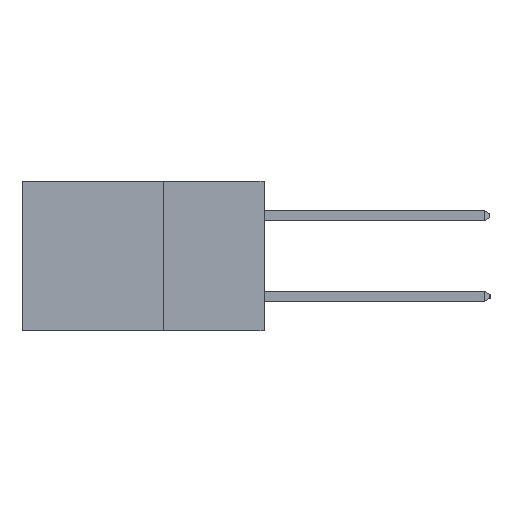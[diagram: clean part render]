
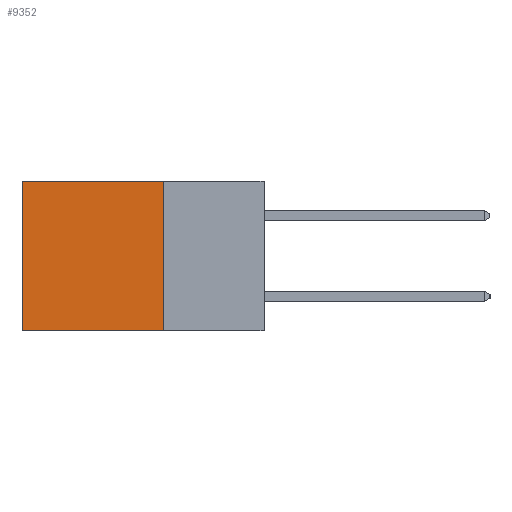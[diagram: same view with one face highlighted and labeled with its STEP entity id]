
A CAD part, left-side view. The second image highlights one B-rep face of the part: STEP entity #9352.
In plain terms, the highlighted planar face has unit normal (-1, 0, 0).
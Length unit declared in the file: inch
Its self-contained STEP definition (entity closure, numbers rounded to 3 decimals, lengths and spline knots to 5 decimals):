
#317 = FACE_OUTER_BOUND ( 'NONE', #8357, .T. ) ;
#375 = VERTEX_POINT ( 'NONE', #10325 ) ;
#2119 = DIRECTION ( 'NONE',  ( 0., 0., -1. ) ) ;
#2528 = CARTESIAN_POINT ( 'NONE',  ( 0.2615, 0.6, 0. ) ) ;
#2644 = AXIS2_PLACEMENT_3D ( 'NONE', #24282, #14203, #2119 ) ;
#3995 = VECTOR ( 'NONE', #12560, 39.37008 ) ;
#4110 = CARTESIAN_POINT ( 'NONE',  ( 0.2615, 0.25, -0.37 ) ) ;
#4550 = CARTESIAN_POINT ( 'NONE',  ( 0.2615, 0.25, 0. ) ) ;
#4869 = CARTESIAN_POINT ( 'NONE',  ( 0.2615, 0.6, -0.37 ) ) ;
#5446 = DIRECTION ( 'NONE',  ( 0., 0., -1. ) ) ;
#7671 = VECTOR ( 'NONE', #8162, 39.37008 ) ;
#7689 = ORIENTED_EDGE ( 'NONE', *, *, #18068, .F. ) ;
#7839 = EDGE_CURVE ( 'NONE', #10593, #375, #9635, .T. ) ;
#8162 = DIRECTION ( 'NONE',  ( 0., 1., 0. ) ) ;
#8357 = EDGE_LOOP ( 'NONE', ( #16962, #7689, #9791, #23721 ) ) ;
#9352 = ADVANCED_FACE ( 'NONE', ( #317 ), #10147, .F. ) ;
#9635 = LINE ( 'NONE', #19548, #15001 ) ;
#9791 = ORIENTED_EDGE ( 'NONE', *, *, #7839, .F. ) ;
#10147 = PLANE ( 'NONE',  #2644 ) ;
#10325 = CARTESIAN_POINT ( 'NONE',  ( 0.2615, 0.25, -0.37 ) ) ;
#10593 = VERTEX_POINT ( 'NONE', #17673 ) ;
#12560 = DIRECTION ( 'NONE',  ( 0., 1., 0. ) ) ;
#14203 = DIRECTION ( 'NONE',  ( 1., 0., 0. ) ) ;
#14393 = VERTEX_POINT ( 'NONE', #18225 ) ;
#14737 = LINE ( 'NONE', #4550, #3995 ) ;
#15001 = VECTOR ( 'NONE', #5446, 39.37008 ) ;
#15250 = EDGE_CURVE ( 'NONE', #16538, #14393, #25424, .T. ) ;
#15375 = VECTOR ( 'NONE', #18977, 39.37008 ) ;
#16538 = VERTEX_POINT ( 'NONE', #2528 ) ;
#16962 = ORIENTED_EDGE ( 'NONE', *, *, #15250, .T. ) ;
#17673 = CARTESIAN_POINT ( 'NONE',  ( 0.2615, 0.25, 0. ) ) ;
#18068 = EDGE_CURVE ( 'NONE', #375, #14393, #19039, .T. ) ;
#18225 = CARTESIAN_POINT ( 'NONE',  ( 0.2615, 0.6, -0.37 ) ) ;
#18977 = DIRECTION ( 'NONE',  ( 0., 0., -1. ) ) ;
#19039 = LINE ( 'NONE', #4110, #7671 ) ;
#19548 = CARTESIAN_POINT ( 'NONE',  ( 0.2615, 0.25, -0.37 ) ) ;
#21518 = EDGE_CURVE ( 'NONE', #10593, #16538, #14737, .T. ) ;
#23721 = ORIENTED_EDGE ( 'NONE', *, *, #21518, .T. ) ;
#24282 = CARTESIAN_POINT ( 'NONE',  ( 0.2615, 0.25, -0.37 ) ) ;
#25424 = LINE ( 'NONE', #4869, #15375 ) ;
